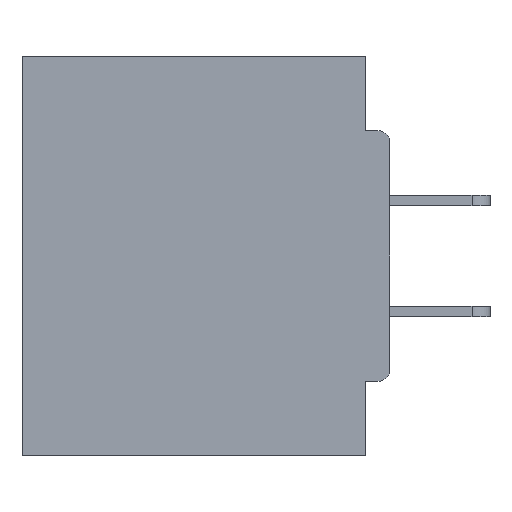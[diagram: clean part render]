
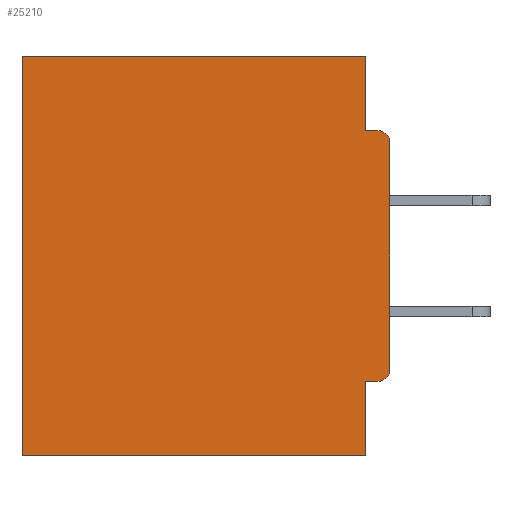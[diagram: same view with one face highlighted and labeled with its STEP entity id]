
A CAD part, left-side view. The second image highlights one B-rep face of the part: STEP entity #25210.
In plain terms, the highlighted planar face has unit normal (-1, 0, 0).
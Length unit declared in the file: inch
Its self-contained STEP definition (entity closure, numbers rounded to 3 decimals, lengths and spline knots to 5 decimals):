
#355 = CARTESIAN_POINT ( 'NONE',  ( 0.298, 0., -0.0935 ) ) ;
#955 = AXIS2_PLACEMENT_3D ( 'NONE', #27186, #12585, #18541 ) ;
#1514 = VERTEX_POINT ( 'NONE', #6513 ) ;
#1982 = ORIENTED_EDGE ( 'NONE', *, *, #16660, .T. ) ;
#2682 = DIRECTION ( 'NONE',  ( 0., 0., -1. ) ) ;
#3030 = LINE ( 'NONE', #8363, #32162 ) ;
#3033 = CARTESIAN_POINT ( 'NONE',  ( 0.298, 0.031, 0. ) ) ;
#3057 = DIRECTION ( 'NONE',  ( 0., 0., -1. ) ) ;
#3664 = VERTEX_POINT ( 'NONE', #21664 ) ;
#3700 = VERTEX_POINT ( 'NONE', #21538 ) ;
#3991 = EDGE_CURVE ( 'NONE', #3664, #14049, #33600, .T. ) ;
#4041 = DIRECTION ( 'NONE',  ( -1., 0., 0. ) ) ;
#5022 = CIRCLE ( 'NONE', #36256, 0.015 ) ;
#5660 = EDGE_CURVE ( 'NONE', #13582, #1514, #24180, .T. ) ;
#6431 = CARTESIAN_POINT ( 'NONE',  ( 0.298, 0.015, -0.4065 ) ) ;
#6513 = CARTESIAN_POINT ( 'NONE',  ( 0.298, 0., -0.3915 ) ) ;
#7739 = ORIENTED_EDGE ( 'NONE', *, *, #20739, .T. ) ;
#8363 = CARTESIAN_POINT ( 'NONE',  ( 0.298, 0.031, -0.5 ) ) ;
#8579 = ORIENTED_EDGE ( 'NONE', *, *, #24129, .F. ) ;
#9332 = EDGE_CURVE ( 'NONE', #36693, #34876, #14193, .T. ) ;
#9461 = VERTEX_POINT ( 'NONE', #3033 ) ;
#11620 = CARTESIAN_POINT ( 'NONE',  ( 0.298, 0., 0. ) ) ;
#11655 = VECTOR ( 'NONE', #35317, 39.37008 ) ;
#12585 = DIRECTION ( 'NONE',  ( 1., 0., 0. ) ) ;
#13062 = DIRECTION ( 'NONE',  ( 0., 0., -1. ) ) ;
#13582 = VERTEX_POINT ( 'NONE', #22686 ) ;
#14049 = VERTEX_POINT ( 'NONE', #23757 ) ;
#14193 = LINE ( 'NONE', #14257, #36894 ) ;
#14257 = CARTESIAN_POINT ( 'NONE',  ( 0.298, 0., -0.4065 ) ) ;
#15174 = DIRECTION ( 'NONE',  ( 0., -1., 0. ) ) ;
#15956 = DIRECTION ( 'NONE',  ( 0., 1., 0. ) ) ;
#16027 = CARTESIAN_POINT ( 'NONE',  ( 0.298, 0.46, 0. ) ) ;
#16244 = VECTOR ( 'NONE', #20613, 39.37008 ) ;
#16335 = CIRCLE ( 'NONE', #19720, 0.015 ) ;
#16380 = EDGE_LOOP ( 'NONE', ( #26538, #17718, #23429, #7739, #1982, #8579, #36572, #38299, #33956, #32549 ) ) ;
#16660 = EDGE_CURVE ( 'NONE', #30473, #3700, #28323, .T. ) ;
#17175 = LINE ( 'NONE', #23708, #16244 ) ;
#17718 = ORIENTED_EDGE ( 'NONE', *, *, #3991, .F. ) ;
#18289 = CARTESIAN_POINT ( 'NONE',  ( 0.298, 0.015, -0.1085 ) ) ;
#18541 = DIRECTION ( 'NONE',  ( 0., 0., -1. ) ) ;
#19500 = EDGE_CURVE ( 'NONE', #9461, #3664, #17175, .T. ) ;
#19720 = AXIS2_PLACEMENT_3D ( 'NONE', #27400, #4041, #13062 ) ;
#20455 = VECTOR ( 'NONE', #21973, 39.37008 ) ;
#20613 = DIRECTION ( 'NONE',  ( 0., 0., -1. ) ) ;
#20739 = EDGE_CURVE ( 'NONE', #9461, #30473, #27756, .T. ) ;
#21538 = CARTESIAN_POINT ( 'NONE',  ( 0.298, 0.46, -0.5 ) ) ;
#21664 = CARTESIAN_POINT ( 'NONE',  ( 0.298, 0.031, -0.0935 ) ) ;
#21745 = CARTESIAN_POINT ( 'NONE',  ( 0.298, 0.46, 0. ) ) ;
#21973 = DIRECTION ( 'NONE',  ( 0., 0., -1. ) ) ;
#22340 = FACE_OUTER_BOUND ( 'NONE', #16380, .T. ) ;
#22686 = CARTESIAN_POINT ( 'NONE',  ( 0.298, 0., -0.1085 ) ) ;
#23153 = DIRECTION ( 'NONE',  ( 0., 1., 0. ) ) ;
#23429 = ORIENTED_EDGE ( 'NONE', *, *, #19500, .F. ) ;
#23708 = CARTESIAN_POINT ( 'NONE',  ( 0.298, 0.031, -0.5 ) ) ;
#23757 = CARTESIAN_POINT ( 'NONE',  ( 0.298, 0.015, -0.0935 ) ) ;
#24034 = VECTOR ( 'NONE', #34832, 39.37008 ) ;
#24129 = EDGE_CURVE ( 'NONE', #30705, #3700, #27074, .T. ) ;
#24180 = LINE ( 'NONE', #11620, #11655 ) ;
#25210 = ADVANCED_FACE ( 'NONE', ( #22340 ), #30310, .F. ) ;
#25671 = VECTOR ( 'NONE', #15174, 39.37008 ) ;
#26538 = ORIENTED_EDGE ( 'NONE', *, *, #28867, .T. ) ;
#26748 = CARTESIAN_POINT ( 'NONE',  ( 0.298, 0.031, -0.5 ) ) ;
#26798 = DIRECTION ( 'NONE',  ( -1., 0., 0. ) ) ;
#27074 = LINE ( 'NONE', #33859, #33584 ) ;
#27186 = CARTESIAN_POINT ( 'NONE',  ( 0.298, 0., 0. ) ) ;
#27400 = CARTESIAN_POINT ( 'NONE',  ( 0.298, 0.015, -0.3915 ) ) ;
#27756 = LINE ( 'NONE', #31824, #24034 ) ;
#28323 = LINE ( 'NONE', #16027, #20455 ) ;
#28867 = EDGE_CURVE ( 'NONE', #13582, #14049, #5022, .T. ) ;
#30310 = PLANE ( 'NONE',  #955 ) ;
#30473 = VERTEX_POINT ( 'NONE', #21745 ) ;
#30705 = VERTEX_POINT ( 'NONE', #26748 ) ;
#31824 = CARTESIAN_POINT ( 'NONE',  ( 0.298, 0., 0. ) ) ;
#32162 = VECTOR ( 'NONE', #2682, 39.37008 ) ;
#32549 = ORIENTED_EDGE ( 'NONE', *, *, #5660, .F. ) ;
#33584 = VECTOR ( 'NONE', #15956, 39.37008 ) ;
#33600 = LINE ( 'NONE', #355, #25671 ) ;
#33859 = CARTESIAN_POINT ( 'NONE',  ( 0.298, 0., -0.5 ) ) ;
#33956 = ORIENTED_EDGE ( 'NONE', *, *, #34224, .T. ) ;
#34224 = EDGE_CURVE ( 'NONE', #36693, #1514, #16335, .T. ) ;
#34832 = DIRECTION ( 'NONE',  ( 0., 1., 0. ) ) ;
#34876 = VERTEX_POINT ( 'NONE', #37557 ) ;
#35317 = DIRECTION ( 'NONE',  ( 0., 0., -1. ) ) ;
#36256 = AXIS2_PLACEMENT_3D ( 'NONE', #18289, #26798, #3057 ) ;
#36572 = ORIENTED_EDGE ( 'NONE', *, *, #36605, .F. ) ;
#36605 = EDGE_CURVE ( 'NONE', #34876, #30705, #3030, .T. ) ;
#36693 = VERTEX_POINT ( 'NONE', #6431 ) ;
#36894 = VECTOR ( 'NONE', #23153, 39.37008 ) ;
#37557 = CARTESIAN_POINT ( 'NONE',  ( 0.298, 0.031, -0.4065 ) ) ;
#38299 = ORIENTED_EDGE ( 'NONE', *, *, #9332, .F. ) ;
